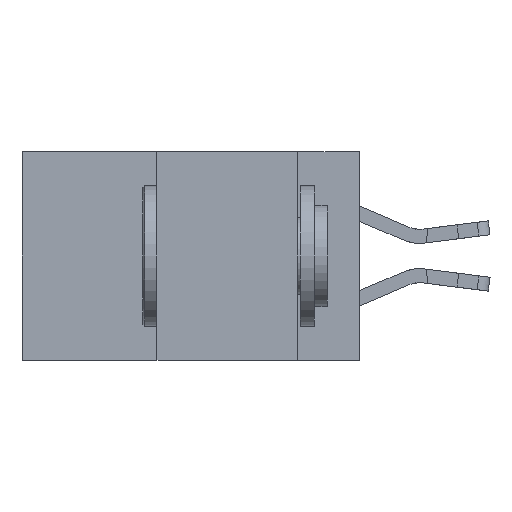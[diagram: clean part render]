
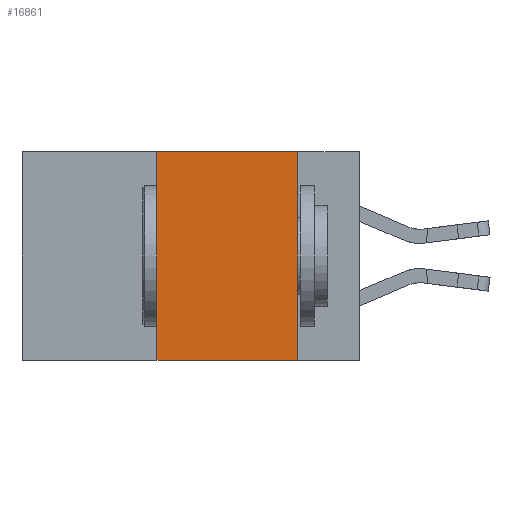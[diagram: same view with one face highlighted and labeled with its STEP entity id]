
A CAD part, left-side view. The second image highlights one B-rep face of the part: STEP entity #16861.
In plain terms, the highlighted planar face has unit normal (-1, 0, 0).
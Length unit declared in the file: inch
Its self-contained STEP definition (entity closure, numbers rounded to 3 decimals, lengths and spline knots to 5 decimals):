
#383 = PLANE ( 'NONE',  #16118 ) ;
#823 = CARTESIAN_POINT ( 'NONE',  ( 0., 0.11, -0.37 ) ) ;
#1777 = EDGE_LOOP ( 'NONE', ( #15605, #8547, #3051, #13931 ) ) ;
#1853 = CARTESIAN_POINT ( 'NONE',  ( 0., 0.11, 0. ) ) ;
#3051 = ORIENTED_EDGE ( 'NONE', *, *, #4029, .F. ) ;
#3375 = DIRECTION ( 'NONE',  ( 0., 0., -1. ) ) ;
#4029 = EDGE_CURVE ( 'NONE', #5537, #9605, #12371, .T. ) ;
#4485 = CARTESIAN_POINT ( 'NONE',  ( 0., 0.36, 0. ) ) ;
#4725 = VECTOR ( 'NONE', #21244, 39.37008 ) ;
#5407 = VECTOR ( 'NONE', #7402, 39.37008 ) ;
#5537 = VERTEX_POINT ( 'NONE', #16664 ) ;
#6198 = DIRECTION ( 'NONE',  ( 0., 0., 1. ) ) ;
#6908 = CARTESIAN_POINT ( 'NONE',  ( 0., 0.11, 0. ) ) ;
#7402 = DIRECTION ( 'NONE',  ( 0., -1., 0. ) ) ;
#8075 = VECTOR ( 'NONE', #3375, 39.37008 ) ;
#8547 = ORIENTED_EDGE ( 'NONE', *, *, #18327, .F. ) ;
#9075 = DIRECTION ( 'NONE',  ( 0., 0., -1. ) ) ;
#9605 = VERTEX_POINT ( 'NONE', #18083 ) ;
#11000 = VECTOR ( 'NONE', #6198, 39.37008 ) ;
#12371 = LINE ( 'NONE', #4485, #11000 ) ;
#12419 = LINE ( 'NONE', #21238, #5407 ) ;
#12676 = CARTESIAN_POINT ( 'NONE',  ( 0., 0.6, 0. ) ) ;
#13931 = ORIENTED_EDGE ( 'NONE', *, *, #13981, .T. ) ;
#13981 = EDGE_CURVE ( 'NONE', #5537, #15425, #12419, .T. ) ;
#14566 = EDGE_CURVE ( 'NONE', #18623, #15425, #14809, .T. ) ;
#14809 = LINE ( 'NONE', #6908, #8075 ) ;
#15425 = VERTEX_POINT ( 'NONE', #823 ) ;
#15605 = ORIENTED_EDGE ( 'NONE', *, *, #14566, .F. ) ;
#15942 = CARTESIAN_POINT ( 'NONE',  ( 0., 0.6, 0. ) ) ;
#16118 = AXIS2_PLACEMENT_3D ( 'NONE', #15942, #17670, #9075 ) ;
#16625 = FACE_OUTER_BOUND ( 'NONE', #1777, .T. ) ;
#16664 = CARTESIAN_POINT ( 'NONE',  ( 0., 0.36, -0.37 ) ) ;
#16861 = ADVANCED_FACE ( 'NONE', ( #16625 ), #383, .F. ) ;
#17377 = LINE ( 'NONE', #12676, #4725 ) ;
#17670 = DIRECTION ( 'NONE',  ( 1., 0., 0. ) ) ;
#18083 = CARTESIAN_POINT ( 'NONE',  ( 0., 0.36, 0. ) ) ;
#18327 = EDGE_CURVE ( 'NONE', #9605, #18623, #17377, .T. ) ;
#18623 = VERTEX_POINT ( 'NONE', #1853 ) ;
#21238 = CARTESIAN_POINT ( 'NONE',  ( 0., 0.6, -0.37 ) ) ;
#21244 = DIRECTION ( 'NONE',  ( 0., -1., 0. ) ) ;
